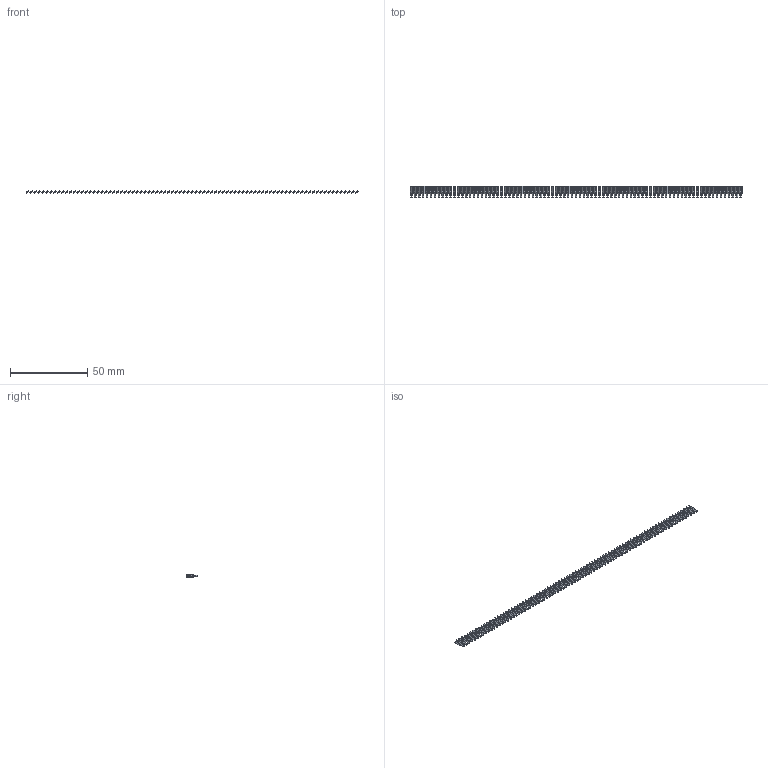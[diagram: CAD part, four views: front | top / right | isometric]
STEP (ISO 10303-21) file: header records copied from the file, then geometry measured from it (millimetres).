
FILE_DESCRIPTION (( 'STEP AP203' ), '1' );
FILE_NAME ('106-085-253-100.STEP', '2020-04-16T22:57:39', ( '' ), ( '' ), 'SwSTEP 2.0', 'SolidWorks 2016', '' );
FILE_SCHEMA (( 'CONFIG_CONTROL_DESIGN' ));
Length unit declared in the file: inch
Products named in the file (2): 100-290-001_100-290-253; 106-085-253-100
Assembly tree (85 placements, depth 2):
  106-085-253-100
    100-290-001_100-290-253  x85
Bounding box: 215.16 x 7.62 x 1.8 mm (x, y, z)
Volume: 469 mm3; surface area: 2924.6 mm2
Topology: 85 solids, 85 shells, 1700 faces, 4590 edges, 3060 vertices
Faces by surface type: plane 1615, cylinder 85
Entity records: 3508 total; most frequent: DIRECTION 272, CARTESIAN_POINT 198, CALENDAR_DATE 180, LOCAL_TIME 180, COORDINATED_UNIVERSAL_TIME_OFFSET 180, DATE_AND_TIME 180, AXIS2_PLACEMENT_3D 110, ORIENTED_EDGE 108
